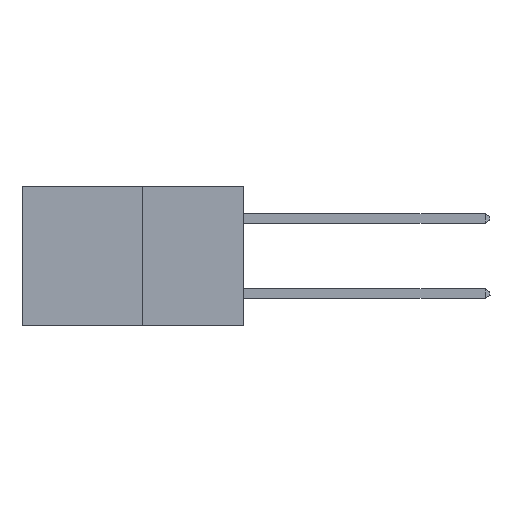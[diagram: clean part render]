
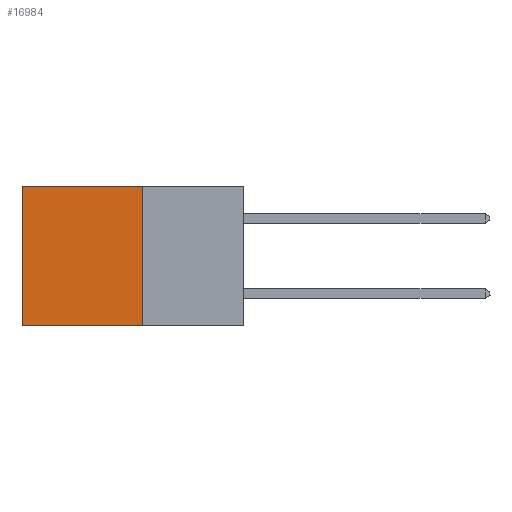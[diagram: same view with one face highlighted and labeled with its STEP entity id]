
A CAD part, left-side view. The second image highlights one B-rep face of the part: STEP entity #16984.
In plain terms, the highlighted planar face has unit normal (-1, 0, 0).
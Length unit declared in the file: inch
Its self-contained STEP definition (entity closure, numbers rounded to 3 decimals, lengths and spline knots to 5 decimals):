
#1029 = CARTESIAN_POINT ( 'NONE',  ( 0.277, 0.27, -0.37 ) ) ;
#1552 = DIRECTION ( 'NONE',  ( 0., 0., -1. ) ) ;
#2478 = EDGE_CURVE ( 'NONE', #10351, #5603, #4112, .T. ) ;
#4112 = LINE ( 'NONE', #10843, #8011 ) ;
#4358 = DIRECTION ( 'NONE',  ( 0., 0., -1. ) ) ;
#4797 = CARTESIAN_POINT ( 'NONE',  ( 0.277, 0.27, -0.37 ) ) ;
#4992 = ORIENTED_EDGE ( 'NONE', *, *, #18240, .F. ) ;
#5077 = LINE ( 'NONE', #9872, #8943 ) ;
#5113 = CARTESIAN_POINT ( 'NONE',  ( 0.277, 0.27, -0.37 ) ) ;
#5172 = FACE_OUTER_BOUND ( 'NONE', #7452, .T. ) ;
#5465 = DIRECTION ( 'NONE',  ( 0., 1., 0. ) ) ;
#5603 = VERTEX_POINT ( 'NONE', #20426 ) ;
#6402 = ORIENTED_EDGE ( 'NONE', *, *, #2478, .T. ) ;
#7452 = EDGE_LOOP ( 'NONE', ( #19602, #4992, #15090, #6402 ) ) ;
#8011 = VECTOR ( 'NONE', #5465, 39.37008 ) ;
#8252 = DIRECTION ( 'NONE',  ( 0., 0., -1. ) ) ;
#8309 = DIRECTION ( 'NONE',  ( 0., 1., 0. ) ) ;
#8683 = CARTESIAN_POINT ( 'NONE',  ( 0.277, 0.27, 0. ) ) ;
#8943 = VECTOR ( 'NONE', #8309, 39.37008 ) ;
#9818 = LINE ( 'NONE', #1029, #13582 ) ;
#9872 = CARTESIAN_POINT ( 'NONE',  ( 0.277, 0.27, -0.37 ) ) ;
#10351 = VERTEX_POINT ( 'NONE', #8683 ) ;
#10843 = CARTESIAN_POINT ( 'NONE',  ( 0.277, 0.27, 0. ) ) ;
#11415 = EDGE_CURVE ( 'NONE', #5603, #14350, #11800, .T. ) ;
#11418 = DIRECTION ( 'NONE',  ( 1., 0., 0. ) ) ;
#11800 = LINE ( 'NONE', #16244, #20035 ) ;
#13582 = VECTOR ( 'NONE', #4358, 39.37008 ) ;
#14350 = VERTEX_POINT ( 'NONE', #16864 ) ;
#14773 = AXIS2_PLACEMENT_3D ( 'NONE', #4797, #11418, #1552 ) ;
#15090 = ORIENTED_EDGE ( 'NONE', *, *, #16779, .F. ) ;
#16244 = CARTESIAN_POINT ( 'NONE',  ( 0.277, 0.59, -0.37 ) ) ;
#16379 = VERTEX_POINT ( 'NONE', #5113 ) ;
#16779 = EDGE_CURVE ( 'NONE', #10351, #16379, #9818, .T. ) ;
#16864 = CARTESIAN_POINT ( 'NONE',  ( 0.277, 0.59, -0.37 ) ) ;
#16984 = ADVANCED_FACE ( 'NONE', ( #5172 ), #19150, .F. ) ;
#18240 = EDGE_CURVE ( 'NONE', #16379, #14350, #5077, .T. ) ;
#19150 = PLANE ( 'NONE',  #14773 ) ;
#19602 = ORIENTED_EDGE ( 'NONE', *, *, #11415, .T. ) ;
#20035 = VECTOR ( 'NONE', #8252, 39.37008 ) ;
#20426 = CARTESIAN_POINT ( 'NONE',  ( 0.277, 0.59, 0. ) ) ;
